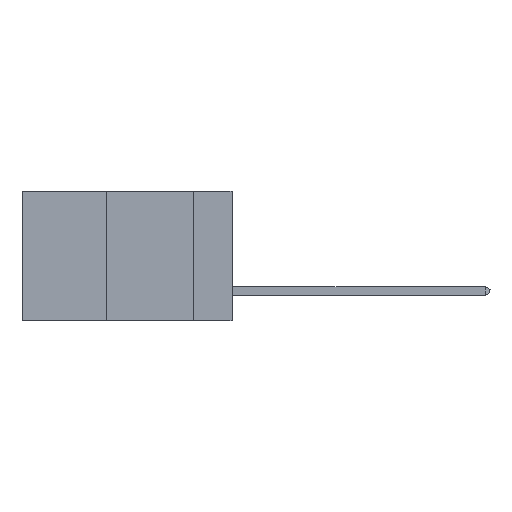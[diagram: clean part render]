
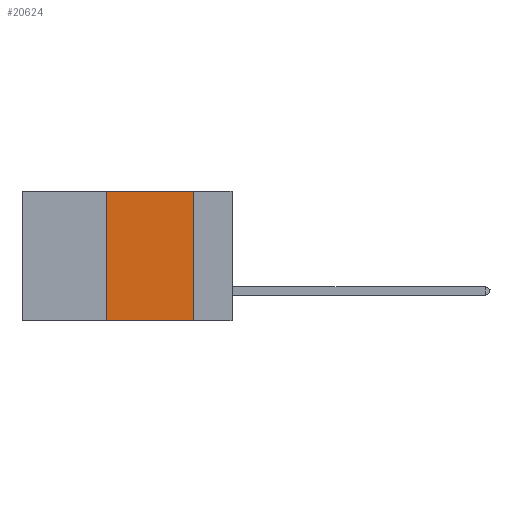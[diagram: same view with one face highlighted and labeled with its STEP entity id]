
A CAD part, left-side view. The second image highlights one B-rep face of the part: STEP entity #20624.
In plain terms, the highlighted planar face has unit normal (-1, 0, 0).
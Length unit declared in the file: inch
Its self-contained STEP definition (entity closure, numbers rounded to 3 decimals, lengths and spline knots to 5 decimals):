
#1934 = DIRECTION ( 'NONE',  ( 0., -1., 0. ) ) ;
#3911 = CARTESIAN_POINT ( 'NONE',  ( 0., 0.36, -0.37 ) ) ;
#4181 = LINE ( 'NONE', #13050, #14550 ) ;
#4248 = CARTESIAN_POINT ( 'NONE',  ( 0., 0.36, 0. ) ) ;
#4576 = ORIENTED_EDGE ( 'NONE', *, *, #19641, .F. ) ;
#5314 = DIRECTION ( 'NONE',  ( 0., 0., -1. ) ) ;
#6016 = VECTOR ( 'NONE', #46528, 39.37008 ) ;
#7770 = DIRECTION ( 'NONE',  ( 0., 0., 1. ) ) ;
#8628 = CARTESIAN_POINT ( 'NONE',  ( 0., 0.11, -0.37 ) ) ;
#9976 = VECTOR ( 'NONE', #28977, 39.37008 ) ;
#11036 = ORIENTED_EDGE ( 'NONE', *, *, #42380, .F. ) ;
#11777 = CARTESIAN_POINT ( 'NONE',  ( 0., 0.36, 0. ) ) ;
#12412 = PLANE ( 'NONE',  #34108 ) ;
#13050 = CARTESIAN_POINT ( 'NONE',  ( 0., 0.6, -0.37 ) ) ;
#13089 = ORIENTED_EDGE ( 'NONE', *, *, #17137, .F. ) ;
#14550 = VECTOR ( 'NONE', #1934, 39.37008 ) ;
#16083 = VECTOR ( 'NONE', #7770, 39.37008 ) ;
#16168 = CARTESIAN_POINT ( 'NONE',  ( 0., 0.11, 0. ) ) ;
#17137 = EDGE_CURVE ( 'NONE', #19197, #36910, #25895, .T. ) ;
#17841 = CARTESIAN_POINT ( 'NONE',  ( 0., 0.6, 0. ) ) ;
#19197 = VERTEX_POINT ( 'NONE', #3911 ) ;
#19641 = EDGE_CURVE ( 'NONE', #36910, #28737, #23882, .T. ) ;
#20612 = EDGE_CURVE ( 'NONE', #19197, #38129, #4181, .T. ) ;
#20624 = ADVANCED_FACE ( 'NONE', ( #41622 ), #12412, .F. ) ;
#20774 = CARTESIAN_POINT ( 'NONE',  ( 0., 0.11, 0. ) ) ;
#21020 = LINE ( 'NONE', #20774, #6016 ) ;
#23882 = LINE ( 'NONE', #17841, #9976 ) ;
#25895 = LINE ( 'NONE', #4248, #16083 ) ;
#28737 = VERTEX_POINT ( 'NONE', #16168 ) ;
#28977 = DIRECTION ( 'NONE',  ( 0., -1., 0. ) ) ;
#31037 = EDGE_LOOP ( 'NONE', ( #11036, #4576, #13089, #41350 ) ) ;
#34108 = AXIS2_PLACEMENT_3D ( 'NONE', #42184, #45913, #5314 ) ;
#36910 = VERTEX_POINT ( 'NONE', #11777 ) ;
#38129 = VERTEX_POINT ( 'NONE', #8628 ) ;
#41350 = ORIENTED_EDGE ( 'NONE', *, *, #20612, .T. ) ;
#41622 = FACE_OUTER_BOUND ( 'NONE', #31037, .T. ) ;
#42184 = CARTESIAN_POINT ( 'NONE',  ( 0., 0.6, 0. ) ) ;
#42380 = EDGE_CURVE ( 'NONE', #28737, #38129, #21020, .T. ) ;
#45913 = DIRECTION ( 'NONE',  ( 1., 0., 0. ) ) ;
#46528 = DIRECTION ( 'NONE',  ( 0., 0., -1. ) ) ;
